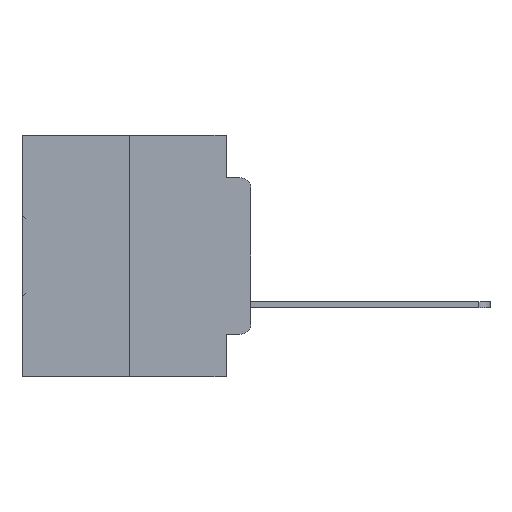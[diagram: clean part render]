
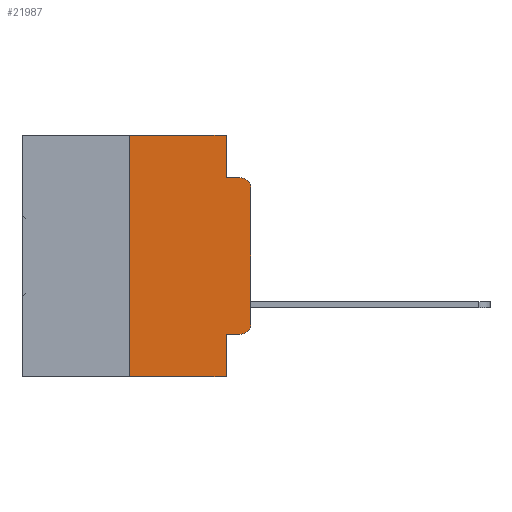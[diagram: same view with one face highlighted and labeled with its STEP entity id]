
A CAD part, left-side view. The second image highlights one B-rep face of the part: STEP entity #21987.
In plain terms, the highlighted planar face has unit normal (-1, 0, 0).
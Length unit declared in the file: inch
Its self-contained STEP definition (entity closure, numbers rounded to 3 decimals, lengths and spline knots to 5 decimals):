
#277 = DIRECTION ( 'NONE',  ( 0., 0., -1. ) ) ;
#1522 = ORIENTED_EDGE ( 'NONE', *, *, #16923, .F. ) ;
#1709 = CARTESIAN_POINT ( 'NONE',  ( 0., 0.25, 0. ) ) ;
#1805 = VECTOR ( 'NONE', #10677, 39.37008 ) ;
#1834 = VECTOR ( 'NONE', #30906, 39.37008 ) ;
#1966 = AXIS2_PLACEMENT_3D ( 'NONE', #32024, #17098, #277 ) ;
#2716 = LINE ( 'NONE', #7889, #1805 ) ;
#2846 = DIRECTION ( 'NONE',  ( 0., -1., 0. ) ) ;
#3365 = AXIS2_PLACEMENT_3D ( 'NONE', #9771, #12477, #30439 ) ;
#3369 = ORIENTED_EDGE ( 'NONE', *, *, #13615, .F. ) ;
#3650 = EDGE_LOOP ( 'NONE', ( #28362, #22635, #1522, #24232, #3369, #11646, #5124, #19760, #20623, #21468 ) ) ;
#3800 = VERTEX_POINT ( 'NONE', #6077 ) ;
#4327 = VERTEX_POINT ( 'NONE', #11752 ) ;
#4682 = CARTESIAN_POINT ( 'NONE',  ( 0., 0.051, -0.5 ) ) ;
#5124 = ORIENTED_EDGE ( 'NONE', *, *, #15102, .T. ) ;
#6077 = CARTESIAN_POINT ( 'NONE',  ( 0., 0., -0.3915 ) ) ;
#7885 = DIRECTION ( 'NONE',  ( 0., -1., 0. ) ) ;
#7889 = CARTESIAN_POINT ( 'NONE',  ( 0., 0.051, 0. ) ) ;
#9771 = CARTESIAN_POINT ( 'NONE',  ( 0., 0.473, 0. ) ) ;
#10677 = DIRECTION ( 'NONE',  ( 0., 0., -1. ) ) ;
#11646 = ORIENTED_EDGE ( 'NONE', *, *, #17079, .F. ) ;
#11752 = CARTESIAN_POINT ( 'NONE',  ( 0., 0.051, -0.4115 ) ) ;
#12329 = LINE ( 'NONE', #27047, #18797 ) ;
#12477 = DIRECTION ( 'NONE',  ( 1., 0., 0. ) ) ;
#12672 = CARTESIAN_POINT ( 'NONE',  ( 0., 0.02, -0.0885 ) ) ;
#12863 = VERTEX_POINT ( 'NONE', #28137 ) ;
#13002 = CARTESIAN_POINT ( 'NONE',  ( 0., 0., 0. ) ) ;
#13351 = VERTEX_POINT ( 'NONE', #32800 ) ;
#13611 = LINE ( 'NONE', #33996, #26693 ) ;
#13615 = EDGE_CURVE ( 'NONE', #26686, #28031, #13611, .T. ) ;
#13626 = LINE ( 'NONE', #23592, #32986 ) ;
#13720 = DIRECTION ( 'NONE',  ( -1., 0., 0. ) ) ;
#14986 = VERTEX_POINT ( 'NONE', #12672 ) ;
#15102 = EDGE_CURVE ( 'NONE', #25218, #24871, #25061, .T. ) ;
#15773 = LINE ( 'NONE', #13002, #1834 ) ;
#15975 = FACE_OUTER_BOUND ( 'NONE', #3650, .T. ) ;
#16859 = EDGE_CURVE ( 'NONE', #3800, #13351, #15773, .T. ) ;
#16904 = EDGE_CURVE ( 'NONE', #13351, #14986, #34071, .T. ) ;
#16923 = EDGE_CURVE ( 'NONE', #24149, #14986, #27851, .T. ) ;
#16967 = EDGE_CURVE ( 'NONE', #28031, #24149, #12329, .T. ) ;
#17079 = EDGE_CURVE ( 'NONE', #25218, #26686, #13626, .T. ) ;
#17098 = DIRECTION ( 'NONE',  ( -1., 0., 0. ) ) ;
#17168 = EDGE_CURVE ( 'NONE', #4327, #24871, #2716, .T. ) ;
#17181 = EDGE_CURVE ( 'NONE', #4327, #12863, #28576, .T. ) ;
#17330 = EDGE_CURVE ( 'NONE', #12863, #3800, #23241, .T. ) ;
#18797 = VECTOR ( 'NONE', #22115, 39.37008 ) ;
#19343 = DIRECTION ( 'NONE',  ( 0., -1., 0. ) ) ;
#19606 = VECTOR ( 'NONE', #19343, 39.37008 ) ;
#19760 = ORIENTED_EDGE ( 'NONE', *, *, #17168, .F. ) ;
#20623 = ORIENTED_EDGE ( 'NONE', *, *, #17181, .T. ) ;
#21468 = ORIENTED_EDGE ( 'NONE', *, *, #17330, .T. ) ;
#21987 = ADVANCED_FACE ( 'NONE', ( #15975 ), #25672, .F. ) ;
#22071 = VECTOR ( 'NONE', #33651, 39.37008 ) ;
#22115 = DIRECTION ( 'NONE',  ( 0., 0., -1. ) ) ;
#22587 = CARTESIAN_POINT ( 'NONE',  ( 0., 0.25, -0.5 ) ) ;
#22635 = ORIENTED_EDGE ( 'NONE', *, *, #16904, .T. ) ;
#23241 = CIRCLE ( 'NONE', #1966, 0.02 ) ;
#23592 = CARTESIAN_POINT ( 'NONE',  ( 0., 0.25, 0. ) ) ;
#24149 = VERTEX_POINT ( 'NONE', #26905 ) ;
#24232 = ORIENTED_EDGE ( 'NONE', *, *, #16967, .F. ) ;
#24432 = CARTESIAN_POINT ( 'NONE',  ( 0., 0.051, -0.0885 ) ) ;
#24578 = CARTESIAN_POINT ( 'NONE',  ( 0., 0.051, 0. ) ) ;
#24871 = VERTEX_POINT ( 'NONE', #4682 ) ;
#25061 = LINE ( 'NONE', #26462, #30656 ) ;
#25218 = VERTEX_POINT ( 'NONE', #22587 ) ;
#25672 = PLANE ( 'NONE',  #3365 ) ;
#26072 = DIRECTION ( 'NONE',  ( 0., 0., 1. ) ) ;
#26462 = CARTESIAN_POINT ( 'NONE',  ( 0., 0.473, -0.5 ) ) ;
#26686 = VERTEX_POINT ( 'NONE', #1709 ) ;
#26693 = VECTOR ( 'NONE', #2846, 39.37008 ) ;
#26905 = CARTESIAN_POINT ( 'NONE',  ( 0., 0.051, -0.0885 ) ) ;
#27047 = CARTESIAN_POINT ( 'NONE',  ( 0., 0.051, 0. ) ) ;
#27851 = LINE ( 'NONE', #24432, #19606 ) ;
#28031 = VERTEX_POINT ( 'NONE', #24578 ) ;
#28137 = CARTESIAN_POINT ( 'NONE',  ( 0., 0.02, -0.4115 ) ) ;
#28362 = ORIENTED_EDGE ( 'NONE', *, *, #16859, .T. ) ;
#28576 = LINE ( 'NONE', #33547, #22071 ) ;
#29133 = CARTESIAN_POINT ( 'NONE',  ( 0., 0.02, -0.1085 ) ) ;
#30439 = DIRECTION ( 'NONE',  ( 0., 0., -1. ) ) ;
#30656 = VECTOR ( 'NONE', #7885, 39.37008 ) ;
#30906 = DIRECTION ( 'NONE',  ( 0., 0., 1. ) ) ;
#31513 = DIRECTION ( 'NONE',  ( 0., 0., -1. ) ) ;
#32024 = CARTESIAN_POINT ( 'NONE',  ( 0., 0.02, -0.3915 ) ) ;
#32130 = AXIS2_PLACEMENT_3D ( 'NONE', #29133, #13720, #31513 ) ;
#32800 = CARTESIAN_POINT ( 'NONE',  ( 0., 0., -0.1085 ) ) ;
#32986 = VECTOR ( 'NONE', #26072, 39.37008 ) ;
#33547 = CARTESIAN_POINT ( 'NONE',  ( 0., 0.051, -0.4115 ) ) ;
#33651 = DIRECTION ( 'NONE',  ( 0., -1., 0. ) ) ;
#33996 = CARTESIAN_POINT ( 'NONE',  ( 0., 0.473, 0. ) ) ;
#34071 = CIRCLE ( 'NONE', #32130, 0.02 ) ;
